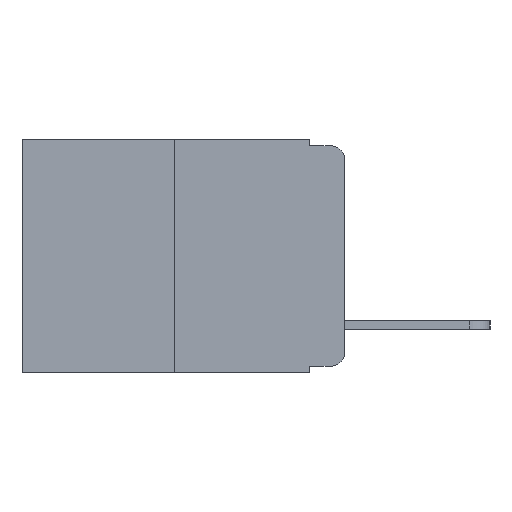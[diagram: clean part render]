
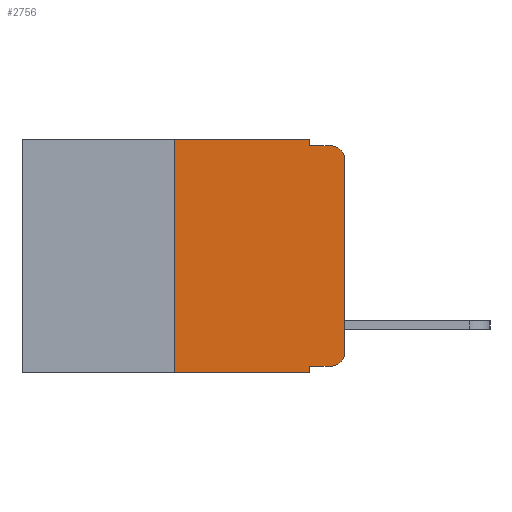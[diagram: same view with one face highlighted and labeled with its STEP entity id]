
A CAD part, left-side view. The second image highlights one B-rep face of the part: STEP entity #2756.
In plain terms, the highlighted planar face has unit normal (-1, 0, 0).
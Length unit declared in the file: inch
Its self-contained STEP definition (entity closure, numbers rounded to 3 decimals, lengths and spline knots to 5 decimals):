
#175 = ORIENTED_EDGE ( 'NONE', *, *, #10399, .F. ) ;
#719 = PLANE ( 'NONE',  #2622 ) ;
#785 = ORIENTED_EDGE ( 'NONE', *, *, #12904, .T. ) ;
#882 = ORIENTED_EDGE ( 'NONE', *, *, #12473, .F. ) ;
#958 = AXIS2_PLACEMENT_3D ( 'NONE', #11990, #6563, #12799 ) ;
#1027 = DIRECTION ( 'NONE',  ( 0., 0., -1. ) ) ;
#1434 = DIRECTION ( 'NONE',  ( 0., 0., -1. ) ) ;
#1544 = ORIENTED_EDGE ( 'NONE', *, *, #12570, .T. ) ;
#1726 = VERTEX_POINT ( 'NONE', #7645 ) ;
#1735 = AXIS2_PLACEMENT_3D ( 'NONE', #5181, #5076, #5025 ) ;
#1776 = VERTEX_POINT ( 'NONE', #4607 ) ;
#1872 = CARTESIAN_POINT ( 'NONE',  ( 0., 0.051, -0.343 ) ) ;
#2150 = CARTESIAN_POINT ( 'NONE',  ( 0., 0.02, -0.333 ) ) ;
#2489 = VERTEX_POINT ( 'NONE', #12858 ) ;
#2622 = AXIS2_PLACEMENT_3D ( 'NONE', #6508, #6266, #1027 ) ;
#2756 = ADVANCED_FACE ( 'NONE', ( #8137 ), #719, .F. ) ;
#2767 = VERTEX_POINT ( 'NONE', #2150 ) ;
#3381 = LINE ( 'NONE', #10936, #6238 ) ;
#3590 = ORIENTED_EDGE ( 'NONE', *, *, #12620, .T. ) ;
#4028 = LINE ( 'NONE', #4849, #6468 ) ;
#4052 = VECTOR ( 'NONE', #10175, 39.37008 ) ;
#4094 = VECTOR ( 'NONE', #8430, 39.37008 ) ;
#4359 = CARTESIAN_POINT ( 'NONE',  ( 0., 0.051, -0.333 ) ) ;
#4455 = DIRECTION ( 'NONE',  ( 0., -1., 0. ) ) ;
#4476 = EDGE_LOOP ( 'NONE', ( #6439, #9401, #9874, #10467, #7995, #175, #785, #882, #1544, #3590 ) ) ;
#4599 = CARTESIAN_POINT ( 'NONE',  ( 0., 0.25, 0. ) ) ;
#4607 = CARTESIAN_POINT ( 'NONE',  ( 0., 0.051, -0.333 ) ) ;
#4849 = CARTESIAN_POINT ( 'NONE',  ( 0., 0.051, -0.01 ) ) ;
#5025 = DIRECTION ( 'NONE',  ( 0., 0., -1. ) ) ;
#5076 = DIRECTION ( 'NONE',  ( -1., 0., 0. ) ) ;
#5181 = CARTESIAN_POINT ( 'NONE',  ( 0., 0.02, -0.03 ) ) ;
#5330 = LINE ( 'NONE', #5512, #12393 ) ;
#5512 = CARTESIAN_POINT ( 'NONE',  ( 0., 0., 0. ) ) ;
#5854 = DIRECTION ( 'NONE',  ( 0., 0., 1. ) ) ;
#6238 = VECTOR ( 'NONE', #10996, 39.37008 ) ;
#6266 = DIRECTION ( 'NONE',  ( 1., 0., 0. ) ) ;
#6437 = CARTESIAN_POINT ( 'NONE',  ( 0., 0.25, -0.343 ) ) ;
#6439 = ORIENTED_EDGE ( 'NONE', *, *, #9209, .T. ) ;
#6468 = VECTOR ( 'NONE', #4455, 39.37008 ) ;
#6508 = CARTESIAN_POINT ( 'NONE',  ( 0., 0.473, 0. ) ) ;
#6563 = DIRECTION ( 'NONE',  ( -1., 0., 0. ) ) ;
#6572 = CARTESIAN_POINT ( 'NONE',  ( 0., 0.051, -0.01 ) ) ;
#6828 = LINE ( 'NONE', #8502, #4094 ) ;
#6909 = CARTESIAN_POINT ( 'NONE',  ( 0., 0.473, -0.343 ) ) ;
#7052 = CIRCLE ( 'NONE', #1735, 0.02 ) ;
#7431 = CARTESIAN_POINT ( 'NONE',  ( 0., 0.02, -0.01 ) ) ;
#7632 = LINE ( 'NONE', #6909, #12154 ) ;
#7645 = CARTESIAN_POINT ( 'NONE',  ( 0., 0., -0.03 ) ) ;
#7816 = DIRECTION ( 'NONE',  ( 0., -1., 0. ) ) ;
#7995 = ORIENTED_EDGE ( 'NONE', *, *, #10764, .F. ) ;
#8137 = FACE_OUTER_BOUND ( 'NONE', #4476, .T. ) ;
#8147 = CARTESIAN_POINT ( 'NONE',  ( 0., 0.051, 0. ) ) ;
#8424 = VECTOR ( 'NONE', #1434, 39.37008 ) ;
#8430 = DIRECTION ( 'NONE',  ( 0., -1., 0. ) ) ;
#8502 = CARTESIAN_POINT ( 'NONE',  ( 0., 0.473, 0. ) ) ;
#8536 = CARTESIAN_POINT ( 'NONE',  ( 0., 0., -0.313 ) ) ;
#8928 = LINE ( 'NONE', #4359, #4052 ) ;
#9209 = EDGE_CURVE ( 'NONE', #10742, #1726, #5330, .T. ) ;
#9293 = EDGE_CURVE ( 'NONE', #1726, #10923, #7052, .T. ) ;
#9312 = EDGE_CURVE ( 'NONE', #11119, #10923, #4028, .T. ) ;
#9401 = ORIENTED_EDGE ( 'NONE', *, *, #9293, .T. ) ;
#9874 = ORIENTED_EDGE ( 'NONE', *, *, #9312, .F. ) ;
#9891 = EDGE_CURVE ( 'NONE', #2489, #11119, #10868, .T. ) ;
#9960 = DIRECTION ( 'NONE',  ( 0., 0., -1. ) ) ;
#10152 = CARTESIAN_POINT ( 'NONE',  ( 0., 0.051, 0. ) ) ;
#10175 = DIRECTION ( 'NONE',  ( 0., -1., 0. ) ) ;
#10399 = EDGE_CURVE ( 'NONE', #11139, #12718, #3381, .T. ) ;
#10429 = LINE ( 'NONE', #8147, #12680 ) ;
#10467 = ORIENTED_EDGE ( 'NONE', *, *, #9891, .F. ) ;
#10742 = VERTEX_POINT ( 'NONE', #8536 ) ;
#10764 = EDGE_CURVE ( 'NONE', #12718, #2489, #6828, .T. ) ;
#10868 = LINE ( 'NONE', #10152, #8424 ) ;
#10923 = VERTEX_POINT ( 'NONE', #7431 ) ;
#10936 = CARTESIAN_POINT ( 'NONE',  ( 0., 0.25, 0. ) ) ;
#10996 = DIRECTION ( 'NONE',  ( 0., 0., 1. ) ) ;
#11085 = CIRCLE ( 'NONE', #958, 0.02 ) ;
#11119 = VERTEX_POINT ( 'NONE', #6572 ) ;
#11139 = VERTEX_POINT ( 'NONE', #6437 ) ;
#11855 = VERTEX_POINT ( 'NONE', #1872 ) ;
#11990 = CARTESIAN_POINT ( 'NONE',  ( 0., 0.02, -0.313 ) ) ;
#12154 = VECTOR ( 'NONE', #7816, 39.37008 ) ;
#12393 = VECTOR ( 'NONE', #5854, 39.37008 ) ;
#12473 = EDGE_CURVE ( 'NONE', #1776, #11855, #10429, .T. ) ;
#12570 = EDGE_CURVE ( 'NONE', #1776, #2767, #8928, .T. ) ;
#12620 = EDGE_CURVE ( 'NONE', #2767, #10742, #11085, .T. ) ;
#12680 = VECTOR ( 'NONE', #9960, 39.37008 ) ;
#12718 = VERTEX_POINT ( 'NONE', #4599 ) ;
#12799 = DIRECTION ( 'NONE',  ( 0., 0., -1. ) ) ;
#12858 = CARTESIAN_POINT ( 'NONE',  ( 0., 0.051, 0. ) ) ;
#12904 = EDGE_CURVE ( 'NONE', #11139, #11855, #7632, .T. ) ;
